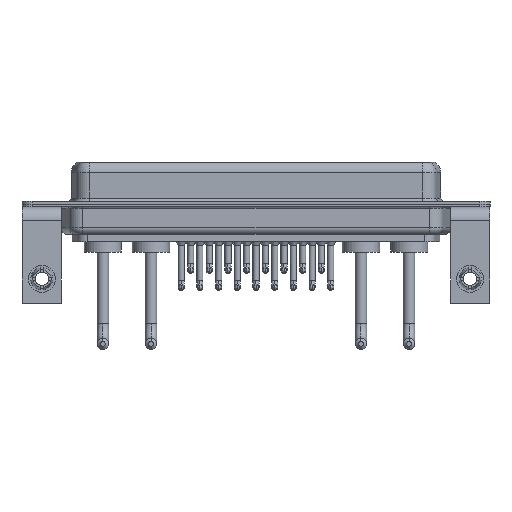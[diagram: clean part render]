
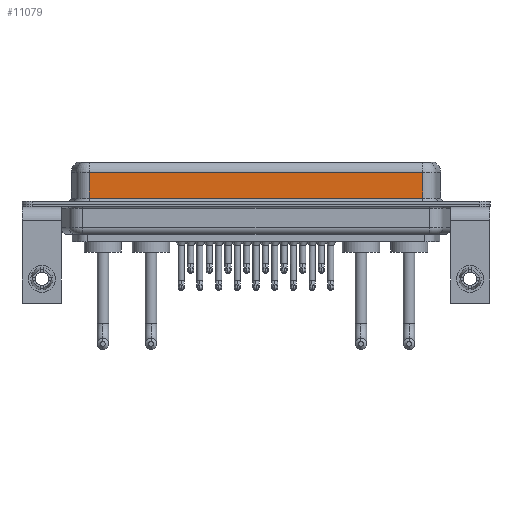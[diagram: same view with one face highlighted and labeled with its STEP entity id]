
A CAD part, front view. The second image highlights one B-rep face of the part: STEP entity #11079.
In plain terms, the highlighted planar face has unit normal (0, -1, 0).
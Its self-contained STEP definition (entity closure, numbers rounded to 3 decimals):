
#359 = EDGE_CURVE ( 'NONE', #17911, #15279, #21726, .T. ) ;
#1011 = DIRECTION ( 'NONE',  ( 0., 1., 0. ) ) ;
#1108 = VECTOR ( 'NONE', #21774, 1000. ) ;
#1985 = LINE ( 'NONE', #17038, #21753 ) ;
#2603 = VERTEX_POINT ( 'NONE', #12603 ) ;
#2788 = LINE ( 'NONE', #8368, #1108 ) ;
#3734 = VECTOR ( 'NONE', #9460, 1000. ) ;
#4921 = EDGE_CURVE ( 'NONE', #17911, #18422, #1985, .T. ) ;
#5794 = EDGE_CURVE ( 'NONE', #15279, #2603, #14996, .T. ) ;
#6661 = EDGE_CURVE ( 'NONE', #2603, #18422, #2788, .T. ) ;
#6715 = FACE_OUTER_BOUND ( 'NONE', #7589, .T. ) ;
#7589 = EDGE_LOOP ( 'NONE', ( #18703, #18297, #9367, #19758 ) ) ;
#7680 = DIRECTION ( 'NONE',  ( 0., 0., -1. ) ) ;
#8368 = CARTESIAN_POINT ( 'NONE',  ( 56.462, -3.95, 0.9 ) ) ;
#8573 = DIRECTION ( 'NONE',  ( 0., 0., 1. ) ) ;
#9367 = ORIENTED_EDGE ( 'NONE', *, *, #5794, .T. ) ;
#9460 = DIRECTION ( 'NONE',  ( 0., 0., -1. ) ) ;
#11079 = ADVANCED_FACE ( 'NONE', ( #6715 ), #23722, .F. ) ;
#11296 = CARTESIAN_POINT ( 'NONE',  ( 7.038, -3.95, 6.4 ) ) ;
#11766 = CARTESIAN_POINT ( 'NONE',  ( 56.462, -3.95, 4.65 ) ) ;
#11950 = CARTESIAN_POINT ( 'NONE',  ( 56.462, -3.95, 0.9 ) ) ;
#12149 = CARTESIAN_POINT ( 'NONE',  ( 56.462, -3.95, 4.65 ) ) ;
#12603 = CARTESIAN_POINT ( 'NONE',  ( 7.038, -3.95, 0.9 ) ) ;
#14462 = VECTOR ( 'NONE', #17672, 1000. ) ;
#14996 = LINE ( 'NONE', #11296, #3734 ) ;
#15279 = VERTEX_POINT ( 'NONE', #15427 ) ;
#15427 = CARTESIAN_POINT ( 'NONE',  ( 7.038, -3.95, 4.65 ) ) ;
#17038 = CARTESIAN_POINT ( 'NONE',  ( 56.462, -3.95, 6.4 ) ) ;
#17672 = DIRECTION ( 'NONE',  ( -1., 0., 0. ) ) ;
#17911 = VERTEX_POINT ( 'NONE', #11766 ) ;
#18297 = ORIENTED_EDGE ( 'NONE', *, *, #359, .T. ) ;
#18422 = VERTEX_POINT ( 'NONE', #11950 ) ;
#18703 = ORIENTED_EDGE ( 'NONE', *, *, #4921, .F. ) ;
#19758 = ORIENTED_EDGE ( 'NONE', *, *, #6661, .T. ) ;
#19763 = CARTESIAN_POINT ( 'NONE',  ( 56.462, -3.95, 6.4 ) ) ;
#20556 = AXIS2_PLACEMENT_3D ( 'NONE', #19763, #1011, #8573 ) ;
#21726 = LINE ( 'NONE', #12149, #14462 ) ;
#21753 = VECTOR ( 'NONE', #7680, 1000. ) ;
#21774 = DIRECTION ( 'NONE',  ( 1., 0., 0. ) ) ;
#23722 = PLANE ( 'NONE',  #20556 ) ;
